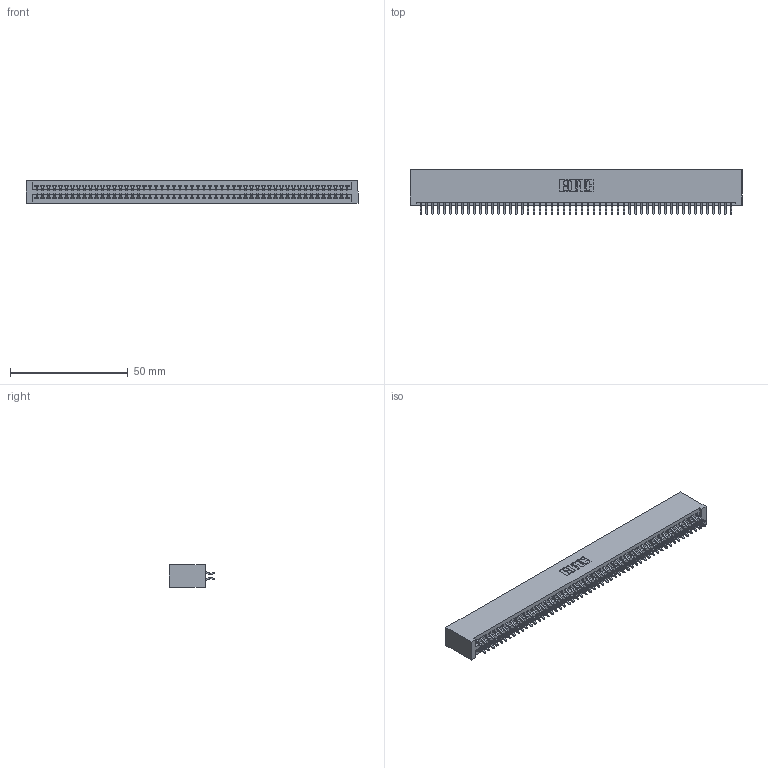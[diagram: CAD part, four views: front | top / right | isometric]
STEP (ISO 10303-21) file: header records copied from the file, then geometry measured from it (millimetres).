
FILE_DESCRIPTION (( 'STEP AP203' ), '1' );
FILE_NAME ('345-106-556-201.STEP', '2018-10-07T03:31:57', ( '' ), ( '' ), 'SwSTEP 2.0', 'SolidWorks 2016', '' );
FILE_SCHEMA (( 'CONFIG_CONTROL_DESIGN' ));
Length unit declared in the file: inch
Products named in the file (3): 345 Part_No Mounting Lugs; 345-292-001_556 Tail; 345-106-556-201
Assembly tree (107 placements, depth 2):
  345-106-556-201
    345 Part_No Mounting Lugs
    345-292-001_556 Tail  x106
Bounding box: 141.22 x 19.24 x 9.4 mm (x, y, z)
Volume: 14432.5 mm3; surface area: 21757.1 mm2
Topology: 107 solids, 107 shells, 6054 faces, 18019 edges, 11870 vertices
Faces by surface type: plane 3998, cylinder 2056
Entity records: 40047 total; most frequent: CARTESIAN_POINT 6716, ORIENTED_EDGE 6638, DIRECTION 5891, EDGE_CURVE 3319, LINE 2975, VECTOR 2975, VERTEX_POINT 2210, AXIS2_PLACEMENT_3D 1458
